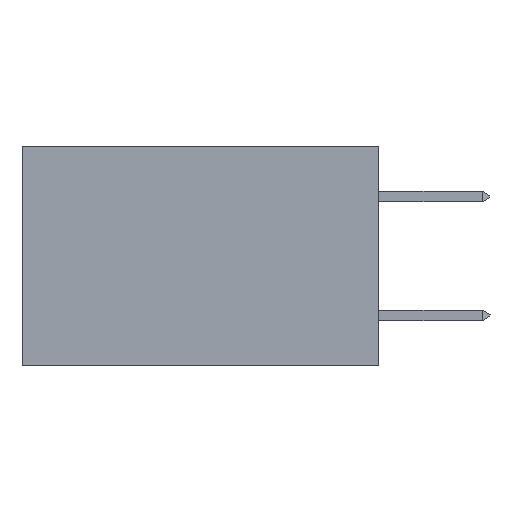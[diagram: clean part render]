
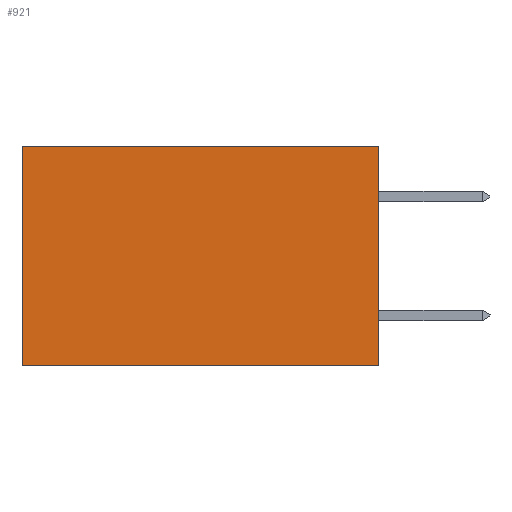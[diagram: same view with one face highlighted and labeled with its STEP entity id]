
A CAD part, left-side view. The second image highlights one B-rep face of the part: STEP entity #921.
In plain terms, the highlighted planar face has unit normal (-1, 0, 0).
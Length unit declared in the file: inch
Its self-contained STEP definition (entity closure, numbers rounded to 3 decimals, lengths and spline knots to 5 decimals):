
#921 = ADVANCED_FACE ( 'NONE', ( #11236 ), #14416, .F. ) ;
#1041 = EDGE_LOOP ( 'NONE', ( #29011, #10372, #6921, #26159 ) ) ;
#1739 = DIRECTION ( 'NONE',  ( 0., 1., 0. ) ) ;
#2933 = DIRECTION ( 'NONE',  ( 0., 0., -1. ) ) ;
#4112 = CARTESIAN_POINT ( 'NONE',  ( 0.298, 0., 0. ) ) ;
#6921 = ORIENTED_EDGE ( 'NONE', *, *, #24241, .F. ) ;
#7268 = LINE ( 'NONE', #21432, #21019 ) ;
#7497 = CARTESIAN_POINT ( 'NONE',  ( 0.298, 0., 0. ) ) ;
#8095 = CARTESIAN_POINT ( 'NONE',  ( 0.298, 0.6, -0.37 ) ) ;
#8192 = CARTESIAN_POINT ( 'NONE',  ( 0.298, 0., -0.37 ) ) ;
#9785 = EDGE_CURVE ( 'NONE', #14263, #27498, #27253, .T. ) ;
#10246 = VERTEX_POINT ( 'NONE', #7497 ) ;
#10372 = ORIENTED_EDGE ( 'NONE', *, *, #9785, .F. ) ;
#11236 = FACE_OUTER_BOUND ( 'NONE', #1041, .T. ) ;
#12157 = EDGE_CURVE ( 'NONE', #10246, #19570, #15372, .T. ) ;
#12302 = DIRECTION ( 'NONE',  ( 0., 1., 0. ) ) ;
#14263 = VERTEX_POINT ( 'NONE', #8192 ) ;
#14416 = PLANE ( 'NONE',  #29175 ) ;
#15372 = LINE ( 'NONE', #4112, #17527 ) ;
#16175 = DIRECTION ( 'NONE',  ( 0., 0., -1. ) ) ;
#16296 = CARTESIAN_POINT ( 'NONE',  ( 0.298, 0.6, 0. ) ) ;
#17527 = VECTOR ( 'NONE', #1739, 39.37008 ) ;
#17727 = EDGE_CURVE ( 'NONE', #19570, #27498, #28425, .T. ) ;
#19160 = CARTESIAN_POINT ( 'NONE',  ( 0.298, 0., 0. ) ) ;
#19570 = VERTEX_POINT ( 'NONE', #16296 ) ;
#21019 = VECTOR ( 'NONE', #23575, 39.37008 ) ;
#21432 = CARTESIAN_POINT ( 'NONE',  ( 0.298, 0., 0. ) ) ;
#23398 = VECTOR ( 'NONE', #16175, 39.37008 ) ;
#23575 = DIRECTION ( 'NONE',  ( 0., 0., -1. ) ) ;
#24241 = EDGE_CURVE ( 'NONE', #10246, #14263, #7268, .T. ) ;
#24334 = CARTESIAN_POINT ( 'NONE',  ( 0.298, 0., -0.37 ) ) ;
#24753 = VECTOR ( 'NONE', #12302, 39.37008 ) ;
#25248 = CARTESIAN_POINT ( 'NONE',  ( 0.298, 0.6, 0. ) ) ;
#26159 = ORIENTED_EDGE ( 'NONE', *, *, #12157, .T. ) ;
#27253 = LINE ( 'NONE', #24334, #24753 ) ;
#27498 = VERTEX_POINT ( 'NONE', #8095 ) ;
#28118 = DIRECTION ( 'NONE',  ( 1., 0., 0. ) ) ;
#28425 = LINE ( 'NONE', #25248, #23398 ) ;
#29011 = ORIENTED_EDGE ( 'NONE', *, *, #17727, .T. ) ;
#29175 = AXIS2_PLACEMENT_3D ( 'NONE', #19160, #28118, #2933 ) ;
